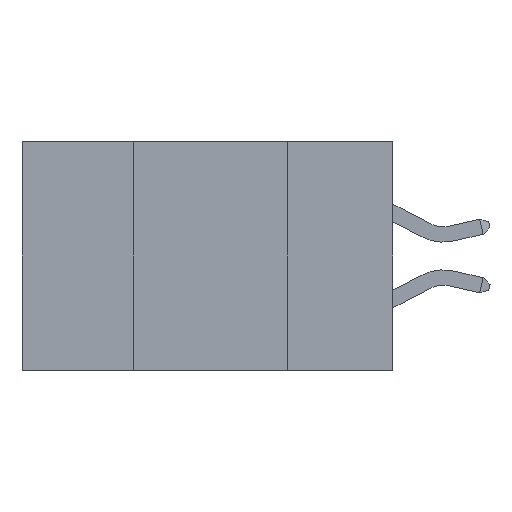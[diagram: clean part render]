
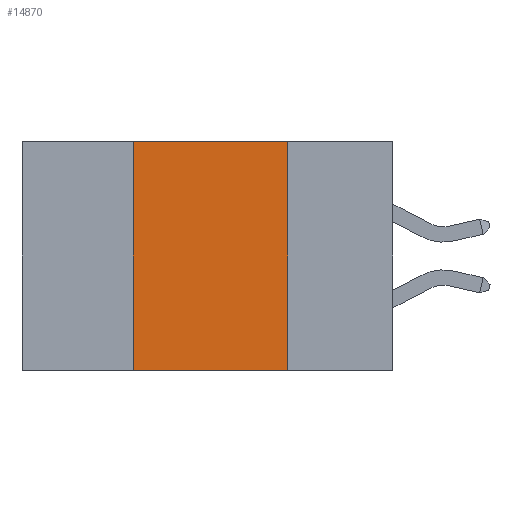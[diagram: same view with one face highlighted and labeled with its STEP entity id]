
A CAD part, left-side view. The second image highlights one B-rep face of the part: STEP entity #14870.
In plain terms, the highlighted planar face has unit normal (-1, 0, 0).
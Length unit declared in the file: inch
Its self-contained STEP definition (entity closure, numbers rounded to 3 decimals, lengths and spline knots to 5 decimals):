
#124 = DIRECTION ( 'NONE',  ( 0., -1., 0. ) ) ;
#866 = CARTESIAN_POINT ( 'NONE',  ( 0., 0.6, 0. ) ) ;
#1441 = ORIENTED_EDGE ( 'NONE', *, *, #8707, .T. ) ;
#2380 = DIRECTION ( 'NONE',  ( 1., 0., 0. ) ) ;
#3662 = LINE ( 'NONE', #23114, #17627 ) ;
#4864 = CARTESIAN_POINT ( 'NONE',  ( 0., 0.42, 0. ) ) ;
#6476 = LINE ( 'NONE', #4864, #6801 ) ;
#6801 = VECTOR ( 'NONE', #23352, 39.37008 ) ;
#7051 = EDGE_CURVE ( 'NONE', #13740, #13960, #8305, .T. ) ;
#7093 = EDGE_CURVE ( 'NONE', #7377, #13740, #16128, .T. ) ;
#7377 = VERTEX_POINT ( 'NONE', #12207 ) ;
#7963 = AXIS2_PLACEMENT_3D ( 'NONE', #10849, #2380, #19146 ) ;
#8305 = LINE ( 'NONE', #23755, #17419 ) ;
#8707 = EDGE_CURVE ( 'NONE', #12843, #13960, #3662, .T. ) ;
#10849 = CARTESIAN_POINT ( 'NONE',  ( 0., 0.6, 0. ) ) ;
#12207 = CARTESIAN_POINT ( 'NONE',  ( 0., 0.42, 0. ) ) ;
#12843 = VERTEX_POINT ( 'NONE', #21502 ) ;
#12917 = ORIENTED_EDGE ( 'NONE', *, *, #7051, .F. ) ;
#13266 = ORIENTED_EDGE ( 'NONE', *, *, #16641, .F. ) ;
#13740 = VERTEX_POINT ( 'NONE', #25263 ) ;
#13960 = VERTEX_POINT ( 'NONE', #21690 ) ;
#14849 = PLANE ( 'NONE',  #7963 ) ;
#14870 = ADVANCED_FACE ( 'NONE', ( #26398 ), #14849, .F. ) ;
#16128 = LINE ( 'NONE', #866, #26391 ) ;
#16641 = EDGE_CURVE ( 'NONE', #12843, #7377, #6476, .T. ) ;
#17419 = VECTOR ( 'NONE', #23675, 39.37008 ) ;
#17627 = VECTOR ( 'NONE', #124, 39.37008 ) ;
#17745 = DIRECTION ( 'NONE',  ( 0., -1., 0. ) ) ;
#19146 = DIRECTION ( 'NONE',  ( 0., 0., -1. ) ) ;
#21502 = CARTESIAN_POINT ( 'NONE',  ( 0., 0.42, -0.37 ) ) ;
#21690 = CARTESIAN_POINT ( 'NONE',  ( 0., 0.17, -0.37 ) ) ;
#23114 = CARTESIAN_POINT ( 'NONE',  ( 0., 0.6, -0.37 ) ) ;
#23352 = DIRECTION ( 'NONE',  ( 0., 0., 1. ) ) ;
#23675 = DIRECTION ( 'NONE',  ( 0., 0., -1. ) ) ;
#23755 = CARTESIAN_POINT ( 'NONE',  ( 0., 0.17, 0. ) ) ;
#24105 = EDGE_LOOP ( 'NONE', ( #12917, #25362, #13266, #1441 ) ) ;
#25263 = CARTESIAN_POINT ( 'NONE',  ( 0., 0.17, 0. ) ) ;
#25362 = ORIENTED_EDGE ( 'NONE', *, *, #7093, .F. ) ;
#26391 = VECTOR ( 'NONE', #17745, 39.37008 ) ;
#26398 = FACE_OUTER_BOUND ( 'NONE', #24105, .T. ) ;
